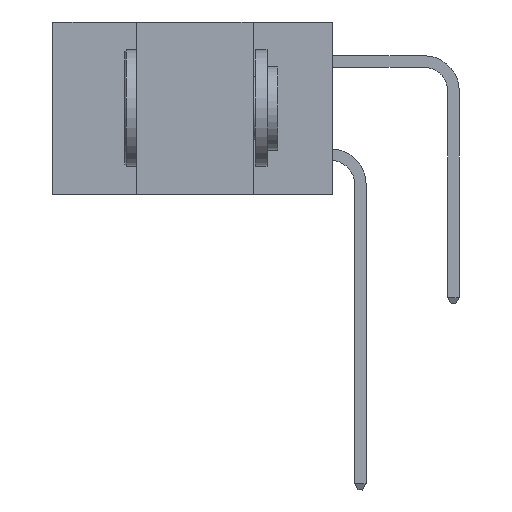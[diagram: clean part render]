
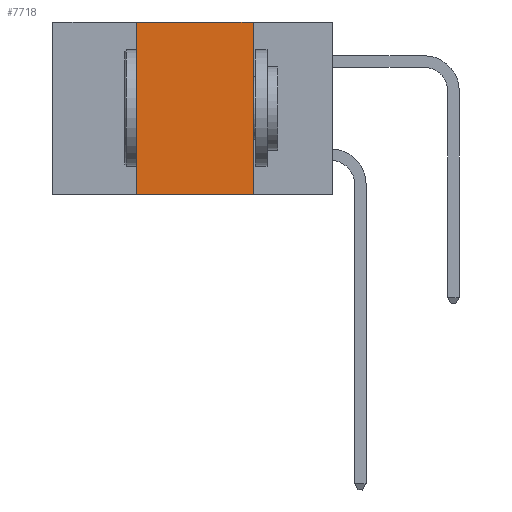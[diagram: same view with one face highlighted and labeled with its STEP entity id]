
A CAD part, left-side view. The second image highlights one B-rep face of the part: STEP entity #7718.
In plain terms, the highlighted planar face has unit normal (-1, 0, 0).
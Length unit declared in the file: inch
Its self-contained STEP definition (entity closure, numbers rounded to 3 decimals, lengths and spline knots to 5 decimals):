
#2043 = CARTESIAN_POINT ( 'NONE',  ( 0., 0.17, 0. ) ) ;
#2083 = CARTESIAN_POINT ( 'NONE',  ( 0., 0.6, 0. ) ) ;
#2575 = ORIENTED_EDGE ( 'NONE', *, *, #4507, .T. ) ;
#2847 = ORIENTED_EDGE ( 'NONE', *, *, #27159, .F. ) ;
#3155 = CARTESIAN_POINT ( 'NONE',  ( 0., 0.17, -0.37 ) ) ;
#3220 = ORIENTED_EDGE ( 'NONE', *, *, #27065, .F. ) ;
#4131 = VERTEX_POINT ( 'NONE', #3155 ) ;
#4507 = EDGE_CURVE ( 'NONE', #20968, #4131, #10468, .T. ) ;
#4771 = LINE ( 'NONE', #2083, #27940 ) ;
#6589 = DIRECTION ( 'NONE',  ( 0., 0., -1. ) ) ;
#7718 = ADVANCED_FACE ( 'NONE', ( #13478 ), #29196, .F. ) ;
#8434 = DIRECTION ( 'NONE',  ( 1., 0., 0. ) ) ;
#10288 = VECTOR ( 'NONE', #6589, 39.37008 ) ;
#10468 = LINE ( 'NONE', #12013, #28935 ) ;
#10661 = LINE ( 'NONE', #27150, #22230 ) ;
#12013 = CARTESIAN_POINT ( 'NONE',  ( 0., 0.6, -0.37 ) ) ;
#13080 = CARTESIAN_POINT ( 'NONE',  ( 0., 0.6, 0. ) ) ;
#13275 = VERTEX_POINT ( 'NONE', #29951 ) ;
#13478 = FACE_OUTER_BOUND ( 'NONE', #13905, .T. ) ;
#13905 = EDGE_LOOP ( 'NONE', ( #2847, #20706, #3220, #2575 ) ) ;
#16727 = DIRECTION ( 'NONE',  ( 0., -1., 0. ) ) ;
#17578 = AXIS2_PLACEMENT_3D ( 'NONE', #13080, #8434, #19924 ) ;
#17600 = CARTESIAN_POINT ( 'NONE',  ( 0., 0.42, -0.37 ) ) ;
#17698 = DIRECTION ( 'NONE',  ( 0., 0., 1. ) ) ;
#19407 = VERTEX_POINT ( 'NONE', #20835 ) ;
#19924 = DIRECTION ( 'NONE',  ( 0., 0., -1. ) ) ;
#20706 = ORIENTED_EDGE ( 'NONE', *, *, #26686, .F. ) ;
#20835 = CARTESIAN_POINT ( 'NONE',  ( 0., 0.17, 0. ) ) ;
#20968 = VERTEX_POINT ( 'NONE', #17600 ) ;
#22230 = VECTOR ( 'NONE', #17698, 39.37008 ) ;
#25355 = DIRECTION ( 'NONE',  ( 0., -1., 0. ) ) ;
#26686 = EDGE_CURVE ( 'NONE', #13275, #19407, #4771, .T. ) ;
#27065 = EDGE_CURVE ( 'NONE', #20968, #13275, #10661, .T. ) ;
#27150 = CARTESIAN_POINT ( 'NONE',  ( 0., 0.42, 0. ) ) ;
#27159 = EDGE_CURVE ( 'NONE', #19407, #4131, #27614, .T. ) ;
#27614 = LINE ( 'NONE', #2043, #10288 ) ;
#27940 = VECTOR ( 'NONE', #25355, 39.37008 ) ;
#28935 = VECTOR ( 'NONE', #16727, 39.37008 ) ;
#29196 = PLANE ( 'NONE',  #17578 ) ;
#29951 = CARTESIAN_POINT ( 'NONE',  ( 0., 0.42, 0. ) ) ;
